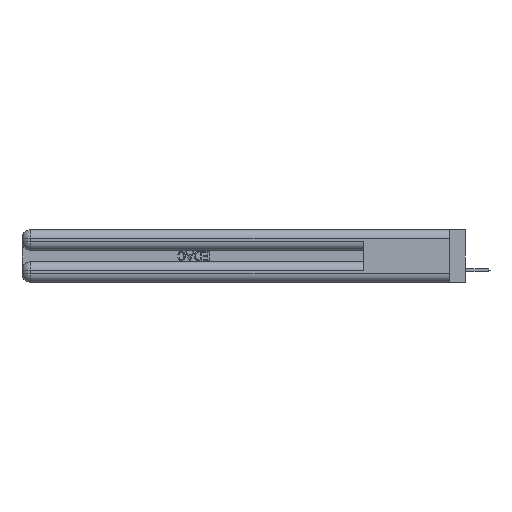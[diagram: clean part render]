
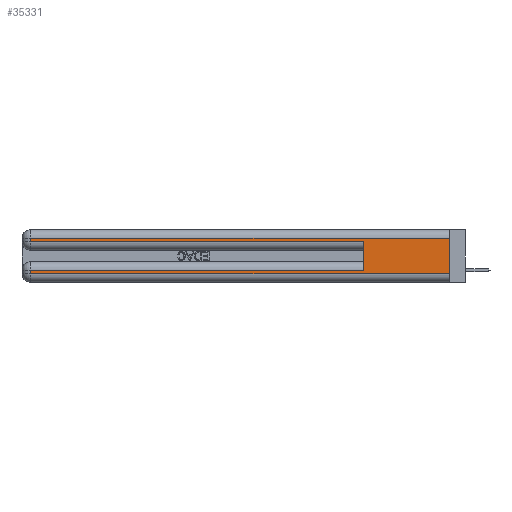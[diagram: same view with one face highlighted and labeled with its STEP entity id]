
A CAD part, left-side view. The second image highlights one B-rep face of the part: STEP entity #35331.
In plain terms, the highlighted planar face has unit normal (-1, 0, 0).
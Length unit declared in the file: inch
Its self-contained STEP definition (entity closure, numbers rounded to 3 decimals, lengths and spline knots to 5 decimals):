
#1277 = DIRECTION ( 'NONE',  ( 0., -1., 0. ) ) ;
#1509 = EDGE_CURVE ( 'NONE', #2565, #22288, #17630, .T. ) ;
#1677 = CARTESIAN_POINT ( 'NONE',  ( 0., 2.94, 0.31 ) ) ;
#1714 = VECTOR ( 'NONE', #22987, 39.37008 ) ;
#2128 = VERTEX_POINT ( 'NONE', #1677 ) ;
#2291 = CARTESIAN_POINT ( 'NONE',  ( 0., 2.94, 0.06 ) ) ;
#2416 = CARTESIAN_POINT ( 'NONE',  ( 0., 0.6, 0.285 ) ) ;
#2499 = EDGE_CURVE ( 'NONE', #2632, #2128, #20989, .T. ) ;
#2565 = VERTEX_POINT ( 'NONE', #41005 ) ;
#2632 = VERTEX_POINT ( 'NONE', #30901 ) ;
#3990 = ORIENTED_EDGE ( 'NONE', *, *, #17811, .T. ) ;
#4336 = DIRECTION ( 'NONE',  ( 0., 1., 0. ) ) ;
#4385 = EDGE_CURVE ( 'NONE', #16696, #32595, #37142, .T. ) ;
#4652 = ORIENTED_EDGE ( 'NONE', *, *, #13873, .T. ) ;
#7236 = VERTEX_POINT ( 'NONE', #32454 ) ;
#8250 = VECTOR ( 'NONE', #43081, 39.37008 ) ;
#10056 = LINE ( 'NONE', #41139, #13452 ) ;
#11631 = CARTESIAN_POINT ( 'NONE',  ( 0., 0.6, 0.145 ) ) ;
#12684 = LINE ( 'NONE', #20249, #23459 ) ;
#13074 = AXIS2_PLACEMENT_3D ( 'NONE', #20887, #31772, #38891 ) ;
#13452 = VECTOR ( 'NONE', #1277, 39.37008 ) ;
#13873 = EDGE_CURVE ( 'NONE', #2565, #16696, #38170, .T. ) ;
#14749 = ORIENTED_EDGE ( 'NONE', *, *, #35059, .T. ) ;
#16476 = VECTOR ( 'NONE', #44275, 39.37008 ) ;
#16598 = DIRECTION ( 'NONE',  ( 0., 0., -1. ) ) ;
#16696 = VERTEX_POINT ( 'NONE', #36439 ) ;
#17630 = LINE ( 'NONE', #11631, #16476 ) ;
#17725 = EDGE_CURVE ( 'NONE', #32595, #40836, #44602, .T. ) ;
#17811 = EDGE_CURVE ( 'NONE', #7236, #22288, #10056, .T. ) ;
#18590 = VECTOR ( 'NONE', #41119, 39.37008 ) ;
#19708 = EDGE_LOOP ( 'NONE', ( #37866, #25411, #14749, #3990, #36921, #4652, #34043, #33772 ) ) ;
#20104 = VECTOR ( 'NONE', #4336, 39.37008 ) ;
#20249 = CARTESIAN_POINT ( 'NONE',  ( 0., 0., 0.37 ) ) ;
#20887 = CARTESIAN_POINT ( 'NONE',  ( 0., 0., 0.37 ) ) ;
#20989 = LINE ( 'NONE', #44508, #1714 ) ;
#21607 = CARTESIAN_POINT ( 'NONE',  ( 0., 0., 0.085 ) ) ;
#21969 = FACE_OUTER_BOUND ( 'NONE', #19708, .T. ) ;
#22288 = VERTEX_POINT ( 'NONE', #2416 ) ;
#22987 = DIRECTION ( 'NONE',  ( 0., 1., 0. ) ) ;
#23459 = VECTOR ( 'NONE', #16598, 39.37008 ) ;
#24157 = CARTESIAN_POINT ( 'NONE',  ( 0., 0., 0.06 ) ) ;
#24911 = EDGE_CURVE ( 'NONE', #2632, #40836, #12684, .T. ) ;
#25411 = ORIENTED_EDGE ( 'NONE', *, *, #2499, .T. ) ;
#27353 = CARTESIAN_POINT ( 'NONE',  ( 0., 0., 0.06 ) ) ;
#30901 = CARTESIAN_POINT ( 'NONE',  ( 0., 0., 0.31 ) ) ;
#31772 = DIRECTION ( 'NONE',  ( 1., 0., 0. ) ) ;
#31798 = CARTESIAN_POINT ( 'NONE',  ( 0., 2.94, 0.37 ) ) ;
#31923 = PLANE ( 'NONE',  #13074 ) ;
#32454 = CARTESIAN_POINT ( 'NONE',  ( 0., 2.94, 0.285 ) ) ;
#32595 = VERTEX_POINT ( 'NONE', #2291 ) ;
#33772 = ORIENTED_EDGE ( 'NONE', *, *, #17725, .T. ) ;
#33803 = CARTESIAN_POINT ( 'NONE',  ( 0., 2.94, 0.37 ) ) ;
#33863 = LINE ( 'NONE', #33803, #18590 ) ;
#34043 = ORIENTED_EDGE ( 'NONE', *, *, #4385, .T. ) ;
#34975 = VECTOR ( 'NONE', #36539, 39.37008 ) ;
#35059 = EDGE_CURVE ( 'NONE', #2128, #7236, #33863, .T. ) ;
#35331 = ADVANCED_FACE ( 'NONE', ( #21969 ), #31923, .F. ) ;
#36439 = CARTESIAN_POINT ( 'NONE',  ( 0., 2.94, 0.085 ) ) ;
#36539 = DIRECTION ( 'NONE',  ( 0., -1., 0. ) ) ;
#36921 = ORIENTED_EDGE ( 'NONE', *, *, #1509, .F. ) ;
#37142 = LINE ( 'NONE', #31798, #8250 ) ;
#37866 = ORIENTED_EDGE ( 'NONE', *, *, #24911, .F. ) ;
#38170 = LINE ( 'NONE', #21607, #20104 ) ;
#38891 = DIRECTION ( 'NONE',  ( 0., 0., -1. ) ) ;
#40836 = VERTEX_POINT ( 'NONE', #27353 ) ;
#41005 = CARTESIAN_POINT ( 'NONE',  ( 0., 0.6, 0.085 ) ) ;
#41119 = DIRECTION ( 'NONE',  ( 0., 0., -1. ) ) ;
#41139 = CARTESIAN_POINT ( 'NONE',  ( 0., 0., 0.285 ) ) ;
#43081 = DIRECTION ( 'NONE',  ( 0., 0., -1. ) ) ;
#44275 = DIRECTION ( 'NONE',  ( 0., 0., 1. ) ) ;
#44508 = CARTESIAN_POINT ( 'NONE',  ( 0., 0., 0.31 ) ) ;
#44602 = LINE ( 'NONE', #24157, #34975 ) ;
